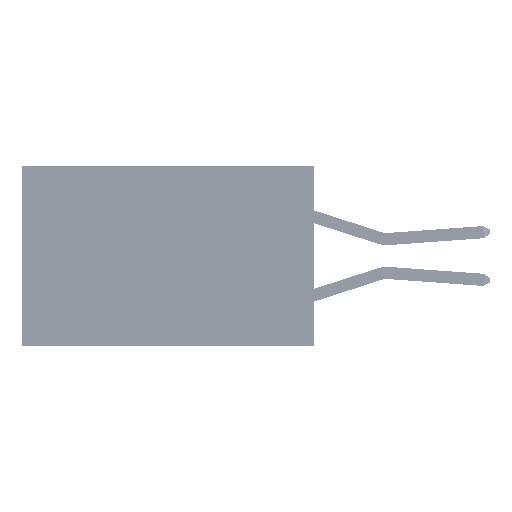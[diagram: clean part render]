
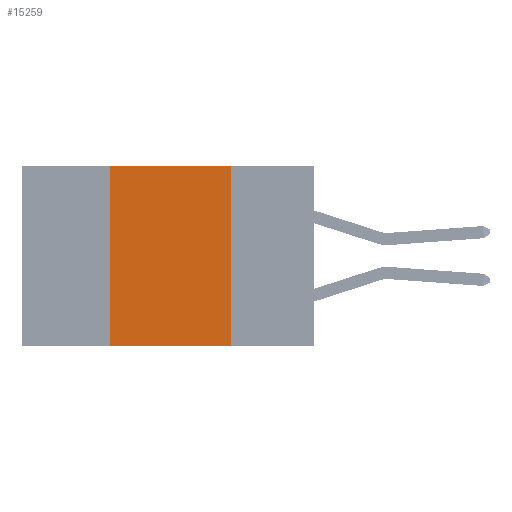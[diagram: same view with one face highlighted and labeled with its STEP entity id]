
A CAD part, left-side view. The second image highlights one B-rep face of the part: STEP entity #15259.
In plain terms, the highlighted planar face has unit normal (-1, 0, 0).
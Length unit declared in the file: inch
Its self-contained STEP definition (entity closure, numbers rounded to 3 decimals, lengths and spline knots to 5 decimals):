
#67 = EDGE_LOOP ( 'NONE', ( #36425, #3456, #21640, #13022 ) ) ;
#1150 = DIRECTION ( 'NONE',  ( 0., 0., -1. ) ) ;
#1464 = DIRECTION ( 'NONE',  ( 0., -1., 0. ) ) ;
#1512 = LINE ( 'NONE', #9353, #32103 ) ;
#2234 = LINE ( 'NONE', #30497, #26430 ) ;
#3456 = ORIENTED_EDGE ( 'NONE', *, *, #11134, .F. ) ;
#4865 = CARTESIAN_POINT ( 'NONE',  ( 0., 0.42, -0.37 ) ) ;
#9093 = FACE_OUTER_BOUND ( 'NONE', #67, .T. ) ;
#9308 = LINE ( 'NONE', #25703, #47874 ) ;
#9353 = CARTESIAN_POINT ( 'NONE',  ( 0., 0.6, -0.37 ) ) ;
#10154 = DIRECTION ( 'NONE',  ( 0., -1., 0. ) ) ;
#11134 = EDGE_CURVE ( 'NONE', #46907, #27336, #9308, .T. ) ;
#12052 = DIRECTION ( 'NONE',  ( 1., 0., 0. ) ) ;
#13022 = ORIENTED_EDGE ( 'NONE', *, *, #52094, .T. ) ;
#13196 = CARTESIAN_POINT ( 'NONE',  ( 0., 0.17, 0. ) ) ;
#15259 = ADVANCED_FACE ( 'NONE', ( #9093 ), #33287, .F. ) ;
#17484 = VECTOR ( 'NONE', #24077, 39.37008 ) ;
#18371 = CARTESIAN_POINT ( 'NONE',  ( 0., 0.17, -0.37 ) ) ;
#20915 = CARTESIAN_POINT ( 'NONE',  ( 0., 0.6, 0. ) ) ;
#21640 = ORIENTED_EDGE ( 'NONE', *, *, #50498, .F. ) ;
#24077 = DIRECTION ( 'NONE',  ( 0., 0., 1. ) ) ;
#25703 = CARTESIAN_POINT ( 'NONE',  ( 0., 0.6, 0. ) ) ;
#26430 = VECTOR ( 'NONE', #1150, 39.37008 ) ;
#27336 = VERTEX_POINT ( 'NONE', #13196 ) ;
#28447 = VERTEX_POINT ( 'NONE', #4865 ) ;
#28638 = LINE ( 'NONE', #36456, #17484 ) ;
#30497 = CARTESIAN_POINT ( 'NONE',  ( 0., 0.17, 0. ) ) ;
#32103 = VECTOR ( 'NONE', #10154, 39.37008 ) ;
#33287 = PLANE ( 'NONE',  #38075 ) ;
#35546 = EDGE_CURVE ( 'NONE', #27336, #45055, #2234, .T. ) ;
#36425 = ORIENTED_EDGE ( 'NONE', *, *, #35546, .F. ) ;
#36456 = CARTESIAN_POINT ( 'NONE',  ( 0., 0.42, 0. ) ) ;
#38075 = AXIS2_PLACEMENT_3D ( 'NONE', #20915, #12052, #41096 ) ;
#41096 = DIRECTION ( 'NONE',  ( 0., 0., -1. ) ) ;
#45055 = VERTEX_POINT ( 'NONE', #18371 ) ;
#46037 = CARTESIAN_POINT ( 'NONE',  ( 0., 0.42, 0. ) ) ;
#46907 = VERTEX_POINT ( 'NONE', #46037 ) ;
#47874 = VECTOR ( 'NONE', #1464, 39.37008 ) ;
#50498 = EDGE_CURVE ( 'NONE', #28447, #46907, #28638, .T. ) ;
#52094 = EDGE_CURVE ( 'NONE', #28447, #45055, #1512, .T. ) ;
